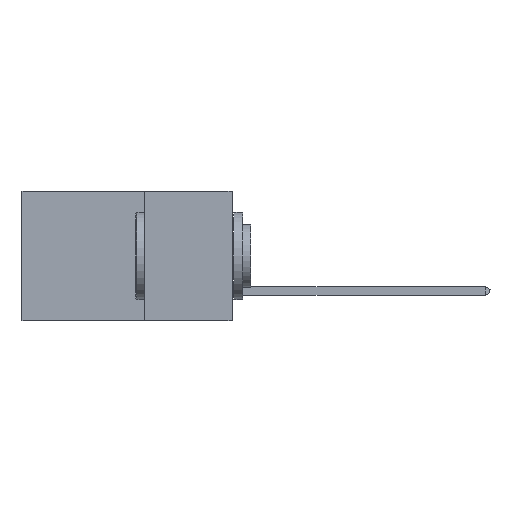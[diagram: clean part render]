
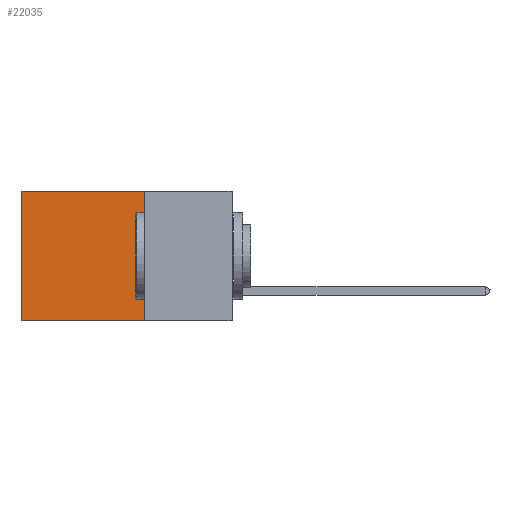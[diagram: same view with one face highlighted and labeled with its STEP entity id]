
A CAD part, left-side view. The second image highlights one B-rep face of the part: STEP entity #22035.
In plain terms, the highlighted planar face has unit normal (-1, 0, 0).
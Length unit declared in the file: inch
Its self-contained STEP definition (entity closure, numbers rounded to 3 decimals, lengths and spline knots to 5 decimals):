
#817 = CARTESIAN_POINT ( 'NONE',  ( 0.2875, 0.25, 0. ) ) ;
#976 = CARTESIAN_POINT ( 'NONE',  ( 0.2875, 0.6, 0. ) ) ;
#1197 = ORIENTED_EDGE ( 'NONE', *, *, #3658, .F. ) ;
#1222 = VECTOR ( 'NONE', #18281, 39.37008 ) ;
#3335 = EDGE_LOOP ( 'NONE', ( #4245, #10735, #1197, #14061 ) ) ;
#3649 = VECTOR ( 'NONE', #3676, 39.37008 ) ;
#3658 = EDGE_CURVE ( 'NONE', #22278, #18425, #8591, .T. ) ;
#3676 = DIRECTION ( 'NONE',  ( 0., 0., -1. ) ) ;
#4245 = ORIENTED_EDGE ( 'NONE', *, *, #15099, .T. ) ;
#4591 = DIRECTION ( 'NONE',  ( 1., 0., 0. ) ) ;
#4677 = LINE ( 'NONE', #17905, #7352 ) ;
#5065 = VERTEX_POINT ( 'NONE', #8888 ) ;
#5190 = DIRECTION ( 'NONE',  ( 0., 1., 0. ) ) ;
#5310 = EDGE_CURVE ( 'NONE', #18425, #5065, #4677, .T. ) ;
#7352 = VECTOR ( 'NONE', #5190, 39.37008 ) ;
#8502 = LINE ( 'NONE', #14380, #1222 ) ;
#8591 = LINE ( 'NONE', #16733, #3649 ) ;
#8888 = CARTESIAN_POINT ( 'NONE',  ( 0.2875, 0.6, -0.37 ) ) ;
#9805 = LINE ( 'NONE', #976, #19250 ) ;
#10735 = ORIENTED_EDGE ( 'NONE', *, *, #5310, .F. ) ;
#13398 = CARTESIAN_POINT ( 'NONE',  ( 0.2875, 0.6, 0. ) ) ;
#13880 = DIRECTION ( 'NONE',  ( 0., 0., -1. ) ) ;
#13960 = PLANE ( 'NONE',  #20912 ) ;
#14061 = ORIENTED_EDGE ( 'NONE', *, *, #17467, .T. ) ;
#14380 = CARTESIAN_POINT ( 'NONE',  ( 0.2875, 0.25, 0. ) ) ;
#15099 = EDGE_CURVE ( 'NONE', #17361, #5065, #9805, .T. ) ;
#16733 = CARTESIAN_POINT ( 'NONE',  ( 0.2875, 0.25, 0. ) ) ;
#17361 = VERTEX_POINT ( 'NONE', #13398 ) ;
#17467 = EDGE_CURVE ( 'NONE', #22278, #17361, #8502, .T. ) ;
#17706 = FACE_OUTER_BOUND ( 'NONE', #3335, .T. ) ;
#17905 = CARTESIAN_POINT ( 'NONE',  ( 0.2875, 0.25, -0.37 ) ) ;
#18281 = DIRECTION ( 'NONE',  ( 0., 1., 0. ) ) ;
#18413 = CARTESIAN_POINT ( 'NONE',  ( 0.2875, 0.25, -0.37 ) ) ;
#18425 = VERTEX_POINT ( 'NONE', #18413 ) ;
#19250 = VECTOR ( 'NONE', #23751, 39.37008 ) ;
#20502 = CARTESIAN_POINT ( 'NONE',  ( 0.2875, 0.25, 0. ) ) ;
#20912 = AXIS2_PLACEMENT_3D ( 'NONE', #817, #4591, #13880 ) ;
#22035 = ADVANCED_FACE ( 'NONE', ( #17706 ), #13960, .F. ) ;
#22278 = VERTEX_POINT ( 'NONE', #20502 ) ;
#23751 = DIRECTION ( 'NONE',  ( 0., 0., -1. ) ) ;
